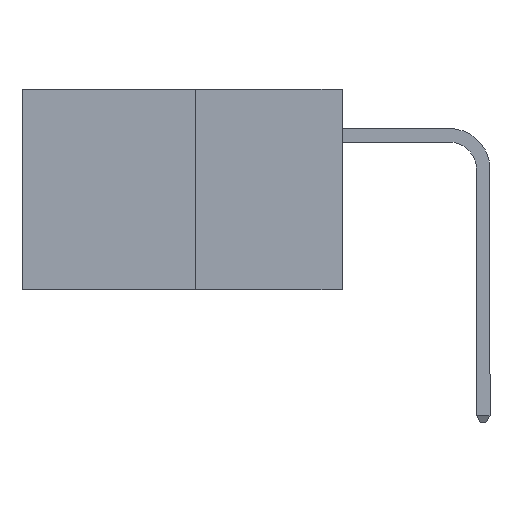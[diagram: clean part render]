
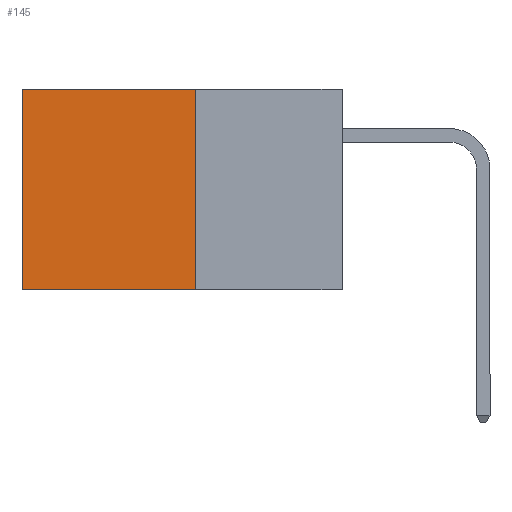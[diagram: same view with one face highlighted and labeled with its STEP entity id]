
A CAD part, left-side view. The second image highlights one B-rep face of the part: STEP entity #145.
In plain terms, the highlighted planar face has unit normal (-1, 0, 0).
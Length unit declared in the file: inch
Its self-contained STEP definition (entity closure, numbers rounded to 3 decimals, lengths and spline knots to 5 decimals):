
#145 = ADVANCED_FACE ( 'NONE', ( #10993 ), #4254, .F. ) ;
#912 = DIRECTION ( 'NONE',  ( 1., 0., 0. ) ) ;
#923 = CARTESIAN_POINT ( 'NONE',  ( 0.277, 0.59, -0.37 ) ) ;
#1188 = CARTESIAN_POINT ( 'NONE',  ( 0.277, 0.27, 0. ) ) ;
#1231 = EDGE_LOOP ( 'NONE', ( #2071, #5155, #5523, #8477 ) ) ;
#1321 = DIRECTION ( 'NONE',  ( 0., 1., 0. ) ) ;
#2071 = ORIENTED_EDGE ( 'NONE', *, *, #2669, .T. ) ;
#2153 = DIRECTION ( 'NONE',  ( 0., 0., -1. ) ) ;
#2385 = AXIS2_PLACEMENT_3D ( 'NONE', #7805, #912, #2153 ) ;
#2669 = EDGE_CURVE ( 'NONE', #14030, #4651, #7049, .T. ) ;
#2674 = DIRECTION ( 'NONE',  ( 0., 1., 0. ) ) ;
#2890 = VECTOR ( 'NONE', #1321, 39.37008 ) ;
#3114 = EDGE_CURVE ( 'NONE', #8072, #4651, #12916, .T. ) ;
#4049 = VECTOR ( 'NONE', #11089, 39.37008 ) ;
#4123 = EDGE_CURVE ( 'NONE', #7103, #14030, #6300, .T. ) ;
#4254 = PLANE ( 'NONE',  #2385 ) ;
#4527 = CARTESIAN_POINT ( 'NONE',  ( 0.277, 0.27, -0.37 ) ) ;
#4651 = VERTEX_POINT ( 'NONE', #9527 ) ;
#5155 = ORIENTED_EDGE ( 'NONE', *, *, #3114, .F. ) ;
#5301 = CARTESIAN_POINT ( 'NONE',  ( 0.277, 0.27, -0.37 ) ) ;
#5523 = ORIENTED_EDGE ( 'NONE', *, *, #13730, .F. ) ;
#6300 = LINE ( 'NONE', #1188, #2890 ) ;
#7049 = LINE ( 'NONE', #923, #4049 ) ;
#7103 = VERTEX_POINT ( 'NONE', #13221 ) ;
#7238 = CARTESIAN_POINT ( 'NONE',  ( 0.277, 0.59, 0. ) ) ;
#7805 = CARTESIAN_POINT ( 'NONE',  ( 0.277, 0.27, -0.37 ) ) ;
#8072 = VERTEX_POINT ( 'NONE', #11800 ) ;
#8477 = ORIENTED_EDGE ( 'NONE', *, *, #4123, .T. ) ;
#9014 = DIRECTION ( 'NONE',  ( 0., 0., -1. ) ) ;
#9271 = LINE ( 'NONE', #4527, #11870 ) ;
#9527 = CARTESIAN_POINT ( 'NONE',  ( 0.277, 0.59, -0.37 ) ) ;
#10002 = VECTOR ( 'NONE', #2674, 39.37008 ) ;
#10993 = FACE_OUTER_BOUND ( 'NONE', #1231, .T. ) ;
#11089 = DIRECTION ( 'NONE',  ( 0., 0., -1. ) ) ;
#11800 = CARTESIAN_POINT ( 'NONE',  ( 0.277, 0.27, -0.37 ) ) ;
#11870 = VECTOR ( 'NONE', #9014, 39.37008 ) ;
#12916 = LINE ( 'NONE', #5301, #10002 ) ;
#13221 = CARTESIAN_POINT ( 'NONE',  ( 0.277, 0.27, 0. ) ) ;
#13730 = EDGE_CURVE ( 'NONE', #7103, #8072, #9271, .T. ) ;
#14030 = VERTEX_POINT ( 'NONE', #7238 ) ;
